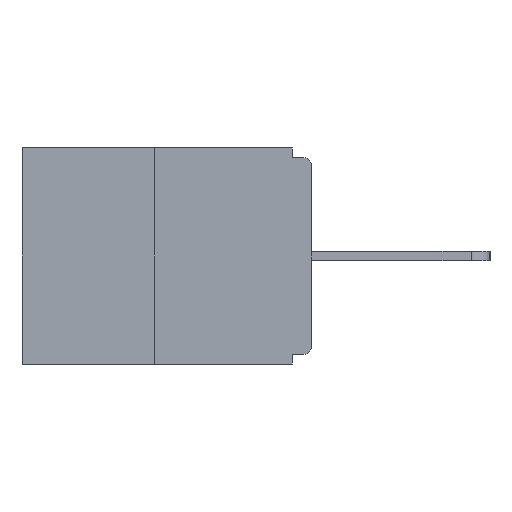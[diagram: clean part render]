
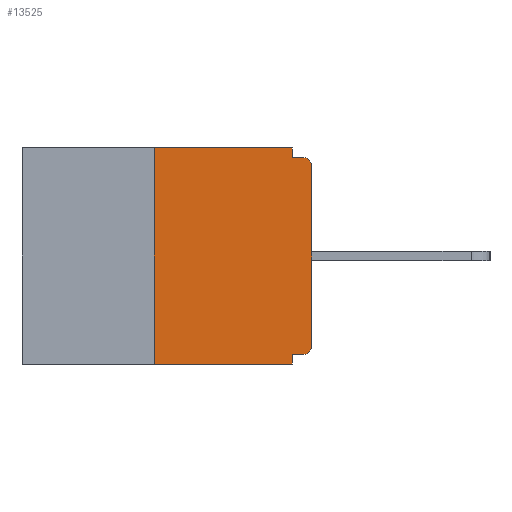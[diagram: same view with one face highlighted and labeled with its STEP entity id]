
A CAD part, left-side view. The second image highlights one B-rep face of the part: STEP entity #13525.
In plain terms, the highlighted planar face has unit normal (-1, 0, 0).
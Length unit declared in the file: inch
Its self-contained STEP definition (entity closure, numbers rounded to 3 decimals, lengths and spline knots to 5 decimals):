
#1 = VECTOR ( 'NONE', #13406, 39.37008 ) ;
#100 = DIRECTION ( 'NONE',  ( 0., 0., -1. ) ) ;
#155 = EDGE_CURVE ( 'NONE', #11487, #4646, #3508, .T. ) ;
#238 = DIRECTION ( 'NONE',  ( 1., 0., 0. ) ) ;
#528 = VERTEX_POINT ( 'NONE', #3267 ) ;
#601 = ORIENTED_EDGE ( 'NONE', *, *, #9682, .T. ) ;
#899 = CARTESIAN_POINT ( 'NONE',  ( 0., 0.031, 0. ) ) ;
#1039 = CARTESIAN_POINT ( 'NONE',  ( 0., 0., -0.328 ) ) ;
#1134 = CIRCLE ( 'NONE', #4083, 0.015 ) ;
#1229 = DIRECTION ( 'NONE',  ( 0., 0., -1. ) ) ;
#1364 = FACE_OUTER_BOUND ( 'NONE', #13026, .T. ) ;
#1504 = ORIENTED_EDGE ( 'NONE', *, *, #5049, .T. ) ;
#2167 = DIRECTION ( 'NONE',  ( 0., 0., -1. ) ) ;
#2202 = LINE ( 'NONE', #7625, #4105 ) ;
#2273 = VECTOR ( 'NONE', #4727, 39.37008 ) ;
#2392 = LINE ( 'NONE', #8026, #2273 ) ;
#2742 = DIRECTION ( 'NONE',  ( 0., 0., -1. ) ) ;
#2817 = VERTEX_POINT ( 'NONE', #10191 ) ;
#2971 = ORIENTED_EDGE ( 'NONE', *, *, #4177, .F. ) ;
#3137 = DIRECTION ( 'NONE',  ( 0., 0., 1. ) ) ;
#3267 = CARTESIAN_POINT ( 'NONE',  ( 0., 0.031, 0. ) ) ;
#3433 = EDGE_CURVE ( 'NONE', #528, #9604, #4307, .T. ) ;
#3478 = ORIENTED_EDGE ( 'NONE', *, *, #3433, .F. ) ;
#3508 = LINE ( 'NONE', #13056, #13908 ) ;
#3810 = DIRECTION ( 'NONE',  ( -1., 0., 0. ) ) ;
#4083 = AXIS2_PLACEMENT_3D ( 'NONE', #5518, #4295, #2167 ) ;
#4105 = VECTOR ( 'NONE', #3137, 39.37008 ) ;
#4177 = EDGE_CURVE ( 'NONE', #10438, #528, #13461, .T. ) ;
#4295 = DIRECTION ( 'NONE',  ( -1., 0., 0. ) ) ;
#4307 = LINE ( 'NONE', #899, #9553 ) ;
#4500 = CARTESIAN_POINT ( 'NONE',  ( 0., 0.25, -0.343 ) ) ;
#4646 = VERTEX_POINT ( 'NONE', #8385 ) ;
#4727 = DIRECTION ( 'NONE',  ( 0., -1., 0. ) ) ;
#4897 = DIRECTION ( 'NONE',  ( 0., 0., 1. ) ) ;
#4975 = CARTESIAN_POINT ( 'NONE',  ( 0., 0.031, -0.015 ) ) ;
#5049 = EDGE_CURVE ( 'NONE', #2817, #11303, #13146, .T. ) ;
#5083 = CARTESIAN_POINT ( 'NONE',  ( 0., 0.015, -0.03 ) ) ;
#5180 = AXIS2_PLACEMENT_3D ( 'NONE', #5083, #3810, #2742 ) ;
#5385 = DIRECTION ( 'NONE',  ( 0., 1., 0. ) ) ;
#5518 = CARTESIAN_POINT ( 'NONE',  ( 0., 0.015, -0.313 ) ) ;
#5769 = CARTESIAN_POINT ( 'NONE',  ( 0., 0.25, 0. ) ) ;
#6544 = DIRECTION ( 'NONE',  ( 0., 0., -1. ) ) ;
#6664 = EDGE_CURVE ( 'NONE', #9604, #11303, #13202, .T. ) ;
#6673 = PLANE ( 'NONE',  #13542 ) ;
#7258 = EDGE_CURVE ( 'NONE', #9014, #11487, #7472, .T. ) ;
#7321 = EDGE_CURVE ( 'NONE', #10637, #4646, #2392, .T. ) ;
#7472 = LINE ( 'NONE', #1039, #13186 ) ;
#7625 = CARTESIAN_POINT ( 'NONE',  ( 0., 0., 0. ) ) ;
#7766 = ORIENTED_EDGE ( 'NONE', *, *, #6664, .F. ) ;
#8026 = CARTESIAN_POINT ( 'NONE',  ( 0., 0.46, -0.343 ) ) ;
#8051 = LINE ( 'NONE', #5769, #8754 ) ;
#8057 = DIRECTION ( 'NONE',  ( 0., -1., 0. ) ) ;
#8268 = CARTESIAN_POINT ( 'NONE',  ( 0., 0.015, -0.015 ) ) ;
#8385 = CARTESIAN_POINT ( 'NONE',  ( 0., 0.031, -0.343 ) ) ;
#8504 = ORIENTED_EDGE ( 'NONE', *, *, #7258, .F. ) ;
#8754 = VECTOR ( 'NONE', #4897, 39.37008 ) ;
#8904 = EDGE_CURVE ( 'NONE', #9014, #11543, #1134, .T. ) ;
#8963 = ORIENTED_EDGE ( 'NONE', *, *, #155, .F. ) ;
#9014 = VERTEX_POINT ( 'NONE', #10060 ) ;
#9085 = ORIENTED_EDGE ( 'NONE', *, *, #12759, .F. ) ;
#9429 = VECTOR ( 'NONE', #8057, 39.37008 ) ;
#9553 = VECTOR ( 'NONE', #6544, 39.37008 ) ;
#9604 = VERTEX_POINT ( 'NONE', #4975 ) ;
#9682 = EDGE_CURVE ( 'NONE', #11543, #2817, #2202, .T. ) ;
#10060 = CARTESIAN_POINT ( 'NONE',  ( 0., 0.015, -0.328 ) ) ;
#10129 = CARTESIAN_POINT ( 'NONE',  ( 0., 0., -0.015 ) ) ;
#10191 = CARTESIAN_POINT ( 'NONE',  ( 0., 0., -0.03 ) ) ;
#10438 = VERTEX_POINT ( 'NONE', #11568 ) ;
#10637 = VERTEX_POINT ( 'NONE', #4500 ) ;
#10972 = CARTESIAN_POINT ( 'NONE',  ( 0., 0.46, 0. ) ) ;
#11303 = VERTEX_POINT ( 'NONE', #8268 ) ;
#11359 = CARTESIAN_POINT ( 'NONE',  ( 0., 0.031, -0.328 ) ) ;
#11487 = VERTEX_POINT ( 'NONE', #11359 ) ;
#11543 = VERTEX_POINT ( 'NONE', #13563 ) ;
#11568 = CARTESIAN_POINT ( 'NONE',  ( 0., 0.25, 0. ) ) ;
#11572 = ORIENTED_EDGE ( 'NONE', *, *, #8904, .T. ) ;
#12759 = EDGE_CURVE ( 'NONE', #10637, #10438, #8051, .T. ) ;
#13026 = EDGE_LOOP ( 'NONE', ( #2971, #9085, #13498, #8963, #8504, #11572, #601, #1504, #7766, #3478 ) ) ;
#13056 = CARTESIAN_POINT ( 'NONE',  ( 0., 0.031, -0.343 ) ) ;
#13146 = CIRCLE ( 'NONE', #5180, 0.015 ) ;
#13186 = VECTOR ( 'NONE', #5385, 39.37008 ) ;
#13202 = LINE ( 'NONE', #10129, #1 ) ;
#13406 = DIRECTION ( 'NONE',  ( 0., -1., 0. ) ) ;
#13461 = LINE ( 'NONE', #13590, #9429 ) ;
#13498 = ORIENTED_EDGE ( 'NONE', *, *, #7321, .T. ) ;
#13525 = ADVANCED_FACE ( 'NONE', ( #1364 ), #6673, .F. ) ;
#13542 = AXIS2_PLACEMENT_3D ( 'NONE', #10972, #238, #1229 ) ;
#13563 = CARTESIAN_POINT ( 'NONE',  ( 0., 0., -0.313 ) ) ;
#13590 = CARTESIAN_POINT ( 'NONE',  ( 0., 0.46, 0. ) ) ;
#13908 = VECTOR ( 'NONE', #100, 39.37008 ) ;
